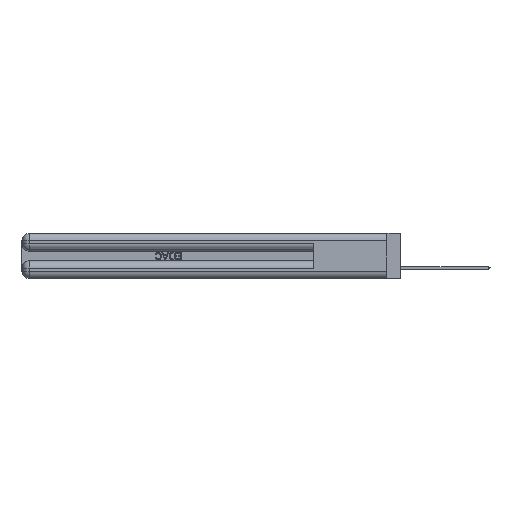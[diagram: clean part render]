
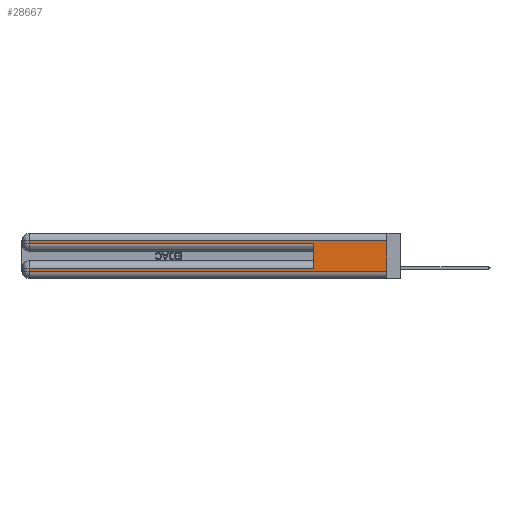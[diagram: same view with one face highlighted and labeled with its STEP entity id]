
A CAD part, left-side view. The second image highlights one B-rep face of the part: STEP entity #28667.
In plain terms, the highlighted planar face has unit normal (-1, 0, 0).
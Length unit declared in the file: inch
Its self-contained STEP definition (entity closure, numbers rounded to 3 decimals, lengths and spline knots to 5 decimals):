
#282 = EDGE_CURVE ( 'NONE', #16369, #12952, #30925, .T. ) ;
#399 = LINE ( 'NONE', #25614, #38850 ) ;
#1272 = CARTESIAN_POINT ( 'NONE',  ( 0., 0.6, 0.145 ) ) ;
#1758 = VERTEX_POINT ( 'NONE', #33128 ) ;
#1877 = CARTESIAN_POINT ( 'NONE',  ( 0., 0., 0.285 ) ) ;
#2851 = CARTESIAN_POINT ( 'NONE',  ( 0., 0., 0.31 ) ) ;
#3849 = CARTESIAN_POINT ( 'NONE',  ( 0., 0., 0.06 ) ) ;
#4998 = LINE ( 'NONE', #3849, #42228 ) ;
#6409 = LINE ( 'NONE', #44397, #26629 ) ;
#6997 = ORIENTED_EDGE ( 'NONE', *, *, #282, .T. ) ;
#7365 = CARTESIAN_POINT ( 'NONE',  ( 0., 2.94, 0.285 ) ) ;
#10207 = LINE ( 'NONE', #1272, #14650 ) ;
#10545 = PLANE ( 'NONE',  #38605 ) ;
#11743 = DIRECTION ( 'NONE',  ( 0., 0., 1. ) ) ;
#12952 = VERTEX_POINT ( 'NONE', #37948 ) ;
#14447 = VERTEX_POINT ( 'NONE', #38686 ) ;
#14650 = VECTOR ( 'NONE', #11743, 39.37008 ) ;
#15543 = DIRECTION ( 'NONE',  ( 0., 1., 0. ) ) ;
#15904 = ORIENTED_EDGE ( 'NONE', *, *, #31228, .T. ) ;
#16369 = VERTEX_POINT ( 'NONE', #7365 ) ;
#17203 = CARTESIAN_POINT ( 'NONE',  ( 0., 2.94, 0.37 ) ) ;
#17440 = DIRECTION ( 'NONE',  ( 0., 0., -1. ) ) ;
#18403 = EDGE_CURVE ( 'NONE', #1758, #16369, #27936, .T. ) ;
#19783 = EDGE_CURVE ( 'NONE', #23517, #36567, #6409, .T. ) ;
#20005 = VERTEX_POINT ( 'NONE', #33268 ) ;
#21598 = LINE ( 'NONE', #41682, #22149 ) ;
#21649 = EDGE_LOOP ( 'NONE', ( #39008, #35910, #35904, #6997, #37634, #42427, #41986, #15904 ) ) ;
#22149 = VECTOR ( 'NONE', #45272, 39.37008 ) ;
#22214 = LINE ( 'NONE', #2851, #25628 ) ;
#23517 = VERTEX_POINT ( 'NONE', #36986 ) ;
#23885 = CARTESIAN_POINT ( 'NONE',  ( 0., 2.94, 0.06 ) ) ;
#24183 = EDGE_CURVE ( 'NONE', #20005, #12952, #10207, .T. ) ;
#24991 = EDGE_CURVE ( 'NONE', #20005, #23517, #399, .T. ) ;
#25547 = FACE_OUTER_BOUND ( 'NONE', #21649, .T. ) ;
#25614 = CARTESIAN_POINT ( 'NONE',  ( 0., 0., 0.085 ) ) ;
#25628 = VECTOR ( 'NONE', #35776, 39.37008 ) ;
#26629 = VECTOR ( 'NONE', #44074, 39.37008 ) ;
#27936 = LINE ( 'NONE', #17203, #38063 ) ;
#28667 = ADVANCED_FACE ( 'NONE', ( #25547 ), #10545, .F. ) ;
#28999 = EDGE_CURVE ( 'NONE', #31700, #14447, #21598, .T. ) ;
#30925 = LINE ( 'NONE', #1877, #43280 ) ;
#31228 = EDGE_CURVE ( 'NONE', #36567, #14447, #4998, .T. ) ;
#31700 = VERTEX_POINT ( 'NONE', #32405 ) ;
#32405 = CARTESIAN_POINT ( 'NONE',  ( 0., 0., 0.31 ) ) ;
#33128 = CARTESIAN_POINT ( 'NONE',  ( 0., 2.94, 0.31 ) ) ;
#33268 = CARTESIAN_POINT ( 'NONE',  ( 0., 0.6, 0.085 ) ) ;
#34845 = DIRECTION ( 'NONE',  ( 0., -1., 0. ) ) ;
#35550 = DIRECTION ( 'NONE',  ( 1., 0., 0. ) ) ;
#35776 = DIRECTION ( 'NONE',  ( 0., 1., 0. ) ) ;
#35904 = ORIENTED_EDGE ( 'NONE', *, *, #18403, .T. ) ;
#35910 = ORIENTED_EDGE ( 'NONE', *, *, #36045, .T. ) ;
#36045 = EDGE_CURVE ( 'NONE', #31700, #1758, #22214, .T. ) ;
#36567 = VERTEX_POINT ( 'NONE', #23885 ) ;
#36986 = CARTESIAN_POINT ( 'NONE',  ( 0., 2.94, 0.085 ) ) ;
#37634 = ORIENTED_EDGE ( 'NONE', *, *, #24183, .F. ) ;
#37948 = CARTESIAN_POINT ( 'NONE',  ( 0., 0.6, 0.285 ) ) ;
#38063 = VECTOR ( 'NONE', #42383, 39.37008 ) ;
#38605 = AXIS2_PLACEMENT_3D ( 'NONE', #39010, #35550, #17440 ) ;
#38686 = CARTESIAN_POINT ( 'NONE',  ( 0., 0., 0.06 ) ) ;
#38850 = VECTOR ( 'NONE', #15543, 39.37008 ) ;
#39008 = ORIENTED_EDGE ( 'NONE', *, *, #28999, .F. ) ;
#39010 = CARTESIAN_POINT ( 'NONE',  ( 0., 0., 0.37 ) ) ;
#41682 = CARTESIAN_POINT ( 'NONE',  ( 0., 0., 0.37 ) ) ;
#41986 = ORIENTED_EDGE ( 'NONE', *, *, #19783, .T. ) ;
#42228 = VECTOR ( 'NONE', #43495, 39.37008 ) ;
#42383 = DIRECTION ( 'NONE',  ( 0., 0., -1. ) ) ;
#42427 = ORIENTED_EDGE ( 'NONE', *, *, #24991, .T. ) ;
#43280 = VECTOR ( 'NONE', #34845, 39.37008 ) ;
#43495 = DIRECTION ( 'NONE',  ( 0., -1., 0. ) ) ;
#44074 = DIRECTION ( 'NONE',  ( 0., 0., -1. ) ) ;
#44397 = CARTESIAN_POINT ( 'NONE',  ( 0., 2.94, 0.37 ) ) ;
#45272 = DIRECTION ( 'NONE',  ( 0., 0., -1. ) ) ;
